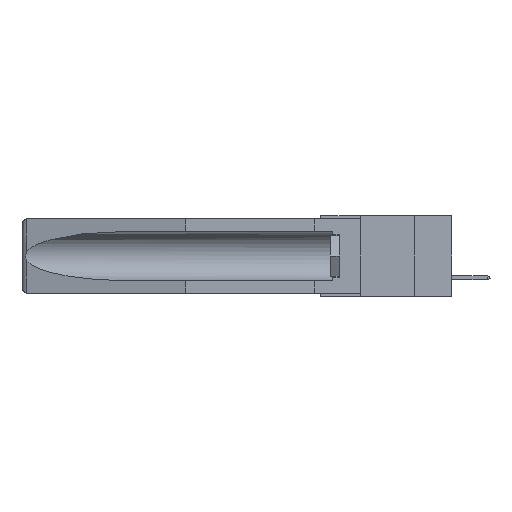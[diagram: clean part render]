
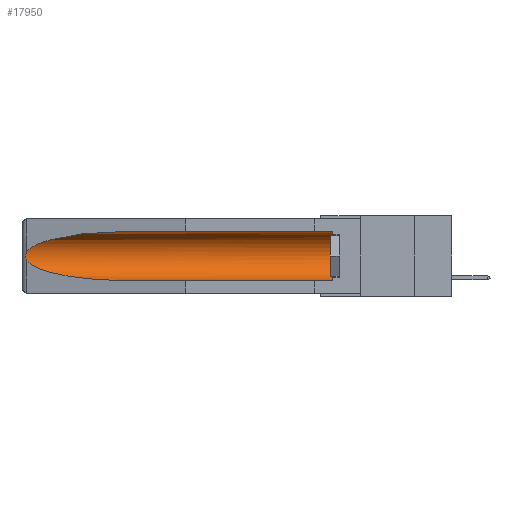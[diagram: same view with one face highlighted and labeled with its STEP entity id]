
A CAD part, left-side view. The second image highlights one B-rep face of the part: STEP entity #17950.
In plain terms, the highlighted cylindrical face has radius 2.857 mm (diameter 5.715 mm), a partial arc.
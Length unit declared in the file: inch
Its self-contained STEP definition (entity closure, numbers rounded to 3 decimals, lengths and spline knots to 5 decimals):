
#954 = VERTEX_POINT ( 'NONE', #7144 ) ;
#1097 = ORIENTED_EDGE ( 'NONE', *, *, #20930, .T. ) ;
#1857 = CARTESIAN_POINT ( 'NONE',  ( 0.155, 1.07973, -0.059 ) ) ;
#2440 =( BOUNDED_CURVE ( )  B_SPLINE_CURVE ( 3, ( #20422, #16008, #24499, #20132 ),
 .UNSPECIFIED., .F., .F. ) 
 B_SPLINE_CURVE_WITH_KNOTS ( ( 4, 4 ),
 ( 0.1948, 1.5708 ),
 .UNSPECIFIED. ) 
 CURVE ( )  GEOMETRIC_REPRESENTATION_ITEM ( )  RATIONAL_B_SPLINE_CURVE ( ( 1., 0.848, 0.848, 1. ) ) 
 REPRESENTATION_ITEM ( '' )  );
#2761 = DIRECTION ( 'NONE',  ( 0., 1., 0. ) ) ;
#3393 = CARTESIAN_POINT ( 'NONE',  ( 0.2675, 1.53308, -0.17534 ) ) ;
#3884 = ORIENTED_EDGE ( 'NONE', *, *, #24997, .T. ) ;
#4320 = CYLINDRICAL_SURFACE ( 'NONE', #25720, 0.1125 ) ;
#4539 = EDGE_CURVE ( 'NONE', #954, #27847, #27153, .T. ) ;
#5578 = VERTEX_POINT ( 'NONE', #14153 ) ;
#7077 = DIRECTION ( 'NONE',  ( 0., 0., 1. ) ) ;
#7144 = CARTESIAN_POINT ( 'NONE',  ( 0.155, 1.07973, -0.059 ) ) ;
#7589 = CARTESIAN_POINT ( 'NONE',  ( 0.26537, 1.52718, -0.14972 ) ) ;
#9384 = CARTESIAN_POINT ( 'NONE',  ( 0.26654, 1.53092, -0.15636 ) ) ;
#9477 = ORIENTED_EDGE ( 'NONE', *, *, #21019, .T. ) ;
#9622 = DIRECTION ( 'NONE',  ( 0., -1., 0. ) ) ;
#9721 = LINE ( 'NONE', #27782, #16353 ) ;
#10980 = VERTEX_POINT ( 'NONE', #17209 ) ;
#11905 = VECTOR ( 'NONE', #2761, 39.37008 ) ;
#12080 = CARTESIAN_POINT ( 'NONE',  ( 0.155, 0.126, -0.284 ) ) ;
#12109 = EDGE_CURVE ( 'NONE', #27847, #5578, #16411, .T. ) ;
#12666 = DIRECTION ( 'NONE',  ( 0., 1., 0. ) ) ;
#12849 = DIRECTION ( 'NONE',  ( 0., 0., 1. ) ) ;
#13266 = AXIS2_PLACEMENT_3D ( 'NONE', #20475, #9622, #7077 ) ;
#14005 = VERTEX_POINT ( 'NONE', #12080 ) ;
#14153 = CARTESIAN_POINT ( 'NONE',  ( 0.26537, 1.52718, -0.19328 ) ) ;
#14644 = CARTESIAN_POINT ( 'NONE',  ( 0.2673, 1.53269, -0.17917 ) ) ;
#16008 = CARTESIAN_POINT ( 'NONE',  ( 0.25451, 1.48313, -0.24835 ) ) ;
#16353 = VECTOR ( 'NONE', #16926, 39.37008 ) ;
#16411 = B_SPLINE_CURVE_WITH_KNOTS ( 'NONE', 3,
 ( #22756, #27548, #9384, #18452, #27254, #3393, #14644, #16783, #16678, #23511 ),
 .UNSPECIFIED., .F., .F.,
 ( 4, 2, 2, 2, 4 ),
 ( 0., 0.00029, 0.00058, 0.00087, 0.00117 ),
 .UNSPECIFIED. ) ;
#16678 = CARTESIAN_POINT ( 'NONE',  ( 0.26597, 1.5296, -0.19026 ) ) ;
#16783 = CARTESIAN_POINT ( 'NONE',  ( 0.26655, 1.53094, -0.18657 ) ) ;
#16926 = DIRECTION ( 'NONE',  ( 0., 1., 0. ) ) ;
#17209 = CARTESIAN_POINT ( 'NONE',  ( 0.155, 1.07973, -0.284 ) ) ;
#17239 = CARTESIAN_POINT ( 'NONE',  ( 0.26537, 1.52718, -0.14972 ) ) ;
#17617 = CARTESIAN_POINT ( 'NONE',  ( 0.21114, 1.30732, -0.059 ) ) ;
#17647 = EDGE_LOOP ( 'NONE', ( #18215, #27894, #3884, #20106, #1097, #9477 ) ) ;
#17950 = ADVANCED_FACE ( 'NONE', ( #25642 ), #4320, .F. ) ;
#18215 = ORIENTED_EDGE ( 'NONE', *, *, #4539, .T. ) ;
#18452 = CARTESIAN_POINT ( 'NONE',  ( 0.2673, 1.5327, -0.16383 ) ) ;
#20106 = ORIENTED_EDGE ( 'NONE', *, *, #25674, .F. ) ;
#20132 = CARTESIAN_POINT ( 'NONE',  ( 0.155, 1.07973, -0.284 ) ) ;
#20422 = CARTESIAN_POINT ( 'NONE',  ( 0.26537, 1.52718, -0.19328 ) ) ;
#20475 = CARTESIAN_POINT ( 'NONE',  ( 0.155, 0.126, -0.1715 ) ) ;
#20930 = EDGE_CURVE ( 'NONE', #14005, #27585, #23020, .T. ) ;
#21019 = EDGE_CURVE ( 'NONE', #27585, #954, #9721, .T. ) ;
#21826 = CARTESIAN_POINT ( 'NONE',  ( 0.155, -0.30754, -0.1715 ) ) ;
#22756 = CARTESIAN_POINT ( 'NONE',  ( 0.26537, 1.52718, -0.14972 ) ) ;
#23020 = CIRCLE ( 'NONE', #13266, 0.1125 ) ;
#23511 = CARTESIAN_POINT ( 'NONE',  ( 0.26537, 1.52718, -0.19328 ) ) ;
#24227 = CARTESIAN_POINT ( 'NONE',  ( 0.25451, 1.48313, -0.09465 ) ) ;
#24380 = CARTESIAN_POINT ( 'NONE',  ( 0.155, 0.126, -0.059 ) ) ;
#24499 = CARTESIAN_POINT ( 'NONE',  ( 0.21114, 1.30732, -0.284 ) ) ;
#24997 = EDGE_CURVE ( 'NONE', #5578, #10980, #2440, .T. ) ;
#25014 = CARTESIAN_POINT ( 'NONE',  ( 0.155, -0.30754, -0.284 ) ) ;
#25642 = FACE_OUTER_BOUND ( 'NONE', #17647, .T. ) ;
#25674 = EDGE_CURVE ( 'NONE', #14005, #10980, #26918, .T. ) ;
#25720 = AXIS2_PLACEMENT_3D ( 'NONE', #21826, #12666, #12849 ) ;
#26918 = LINE ( 'NONE', #25014, #11905 ) ;
#27153 =( BOUNDED_CURVE ( )  B_SPLINE_CURVE ( 3, ( #1857, #17617, #24227, #17239 ),
 .UNSPECIFIED., .F., .F. ) 
 B_SPLINE_CURVE_WITH_KNOTS ( ( 4, 4 ),
 ( 4.71239, 6.08839 ),
 .UNSPECIFIED. ) 
 CURVE ( )  GEOMETRIC_REPRESENTATION_ITEM ( )  RATIONAL_B_SPLINE_CURVE ( ( 1., 0.848, 0.848, 1. ) ) 
 REPRESENTATION_ITEM ( '' )  );
#27254 = CARTESIAN_POINT ( 'NONE',  ( 0.2675, 1.53308, -0.16763 ) ) ;
#27548 = CARTESIAN_POINT ( 'NONE',  ( 0.26597, 1.52961, -0.15275 ) ) ;
#27585 = VERTEX_POINT ( 'NONE', #24380 ) ;
#27782 = CARTESIAN_POINT ( 'NONE',  ( 0.155, -0.30754, -0.059 ) ) ;
#27847 = VERTEX_POINT ( 'NONE', #7589 ) ;
#27894 = ORIENTED_EDGE ( 'NONE', *, *, #12109, .T. ) ;
